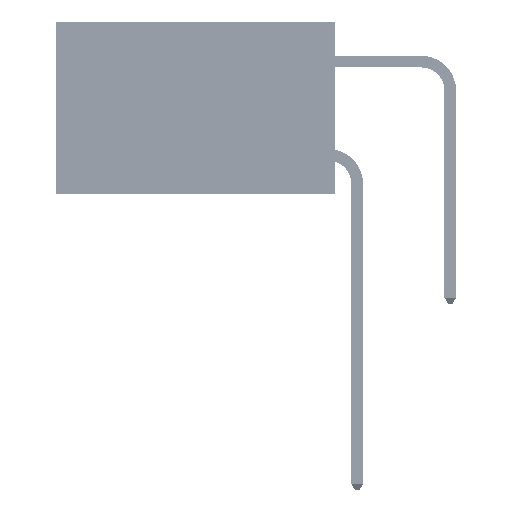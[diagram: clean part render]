
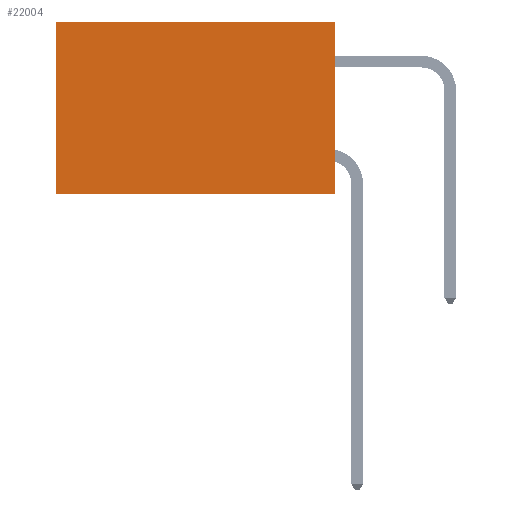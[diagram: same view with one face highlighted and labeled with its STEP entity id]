
A CAD part, left-side view. The second image highlights one B-rep face of the part: STEP entity #22004.
In plain terms, the highlighted planar face has unit normal (-1, 0, 0).
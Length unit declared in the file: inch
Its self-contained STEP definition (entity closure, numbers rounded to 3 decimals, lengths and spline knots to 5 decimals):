
#646 = EDGE_LOOP ( 'NONE', ( #19929, #15307, #42572, #42913 ) ) ;
#5011 = VECTOR ( 'NONE', #37205, 39.37008 ) ;
#7386 = EDGE_CURVE ( 'NONE', #40648, #12884, #35622, .T. ) ;
#8448 = DIRECTION ( 'NONE',  ( 0., 0., -1. ) ) ;
#11078 = CARTESIAN_POINT ( 'NONE',  ( 0.2875, 0.6, 0. ) ) ;
#12884 = VERTEX_POINT ( 'NONE', #35084 ) ;
#14572 = EDGE_CURVE ( 'NONE', #39692, #40648, #22827, .T. ) ;
#14821 = LINE ( 'NONE', #25904, #5011 ) ;
#15307 = ORIENTED_EDGE ( 'NONE', *, *, #7386, .F. ) ;
#17051 = CARTESIAN_POINT ( 'NONE',  ( 0.2875, 0., 0. ) ) ;
#17286 = EDGE_CURVE ( 'NONE', #39692, #24940, #38761, .T. ) ;
#19929 = ORIENTED_EDGE ( 'NONE', *, *, #31510, .T. ) ;
#22004 = ADVANCED_FACE ( 'NONE', ( #24756 ), #45066, .F. ) ;
#22576 = CARTESIAN_POINT ( 'NONE',  ( 0.2875, 0., -0.37 ) ) ;
#22827 = LINE ( 'NONE', #26261, #24009 ) ;
#22884 = CARTESIAN_POINT ( 'NONE',  ( 0.2875, 0., 0. ) ) ;
#24009 = VECTOR ( 'NONE', #41600, 39.37008 ) ;
#24756 = FACE_OUTER_BOUND ( 'NONE', #646, .T. ) ;
#24940 = VERTEX_POINT ( 'NONE', #11078 ) ;
#25056 = DIRECTION ( 'NONE',  ( 0., 1., 0. ) ) ;
#25215 = VECTOR ( 'NONE', #26338, 39.37008 ) ;
#25904 = CARTESIAN_POINT ( 'NONE',  ( 0.2875, 0.6, 0. ) ) ;
#26261 = CARTESIAN_POINT ( 'NONE',  ( 0.2875, 0., 0. ) ) ;
#26338 = DIRECTION ( 'NONE',  ( 0., 1., 0. ) ) ;
#26632 = DIRECTION ( 'NONE',  ( 1., 0., 0. ) ) ;
#31510 = EDGE_CURVE ( 'NONE', #24940, #12884, #14821, .T. ) ;
#35084 = CARTESIAN_POINT ( 'NONE',  ( 0.2875, 0.6, -0.37 ) ) ;
#35622 = LINE ( 'NONE', #22576, #25215 ) ;
#37164 = CARTESIAN_POINT ( 'NONE',  ( 0.2875, 0., 0. ) ) ;
#37205 = DIRECTION ( 'NONE',  ( 0., 0., -1. ) ) ;
#38761 = LINE ( 'NONE', #17051, #47468 ) ;
#39692 = VERTEX_POINT ( 'NONE', #37164 ) ;
#40648 = VERTEX_POINT ( 'NONE', #46652 ) ;
#41600 = DIRECTION ( 'NONE',  ( 0., 0., -1. ) ) ;
#42572 = ORIENTED_EDGE ( 'NONE', *, *, #14572, .F. ) ;
#42913 = ORIENTED_EDGE ( 'NONE', *, *, #17286, .T. ) ;
#45066 = PLANE ( 'NONE',  #46409 ) ;
#46409 = AXIS2_PLACEMENT_3D ( 'NONE', #22884, #26632, #8448 ) ;
#46652 = CARTESIAN_POINT ( 'NONE',  ( 0.2875, 0., -0.37 ) ) ;
#47468 = VECTOR ( 'NONE', #25056, 39.37008 ) ;
